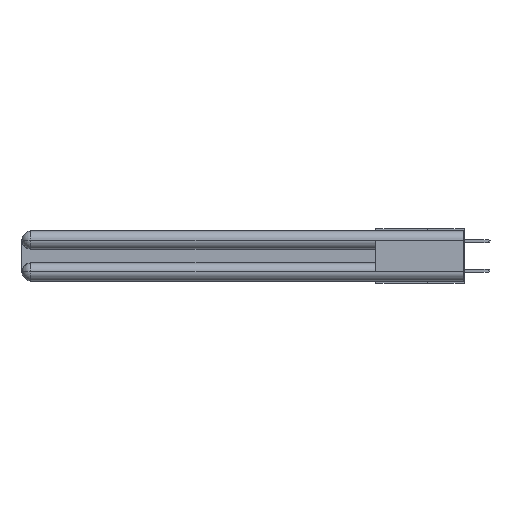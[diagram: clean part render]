
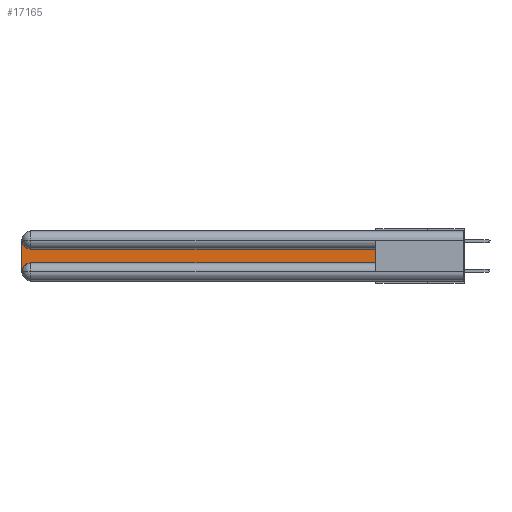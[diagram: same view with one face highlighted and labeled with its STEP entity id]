
A CAD part, left-side view. The second image highlights one B-rep face of the part: STEP entity #17165.
In plain terms, the highlighted planar face has unit normal (-1, 0, 0).
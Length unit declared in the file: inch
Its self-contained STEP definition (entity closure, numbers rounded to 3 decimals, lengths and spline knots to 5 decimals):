
#747 = CARTESIAN_POINT ( 'NONE',  ( 0.075, 0.6, -0.2175 ) ) ;
#974 = VERTEX_POINT ( 'NONE', #21450 ) ;
#1210 = EDGE_CURVE ( 'NONE', #27444, #25030, #19799, .T. ) ;
#1501 = VECTOR ( 'NONE', #4191, 39.37008 ) ;
#1812 = CARTESIAN_POINT ( 'NONE',  ( 0.075, 3., -0.2175 ) ) ;
#1838 = CARTESIAN_POINT ( 'NONE',  ( 0.075, 0.6, -0.2175 ) ) ;
#2228 = VERTEX_POINT ( 'NONE', #24825 ) ;
#2661 = AXIS2_PLACEMENT_3D ( 'NONE', #15143, #6917, #24907 ) ;
#3260 = DIRECTION ( 'NONE',  ( 0., -1., 0. ) ) ;
#4191 = DIRECTION ( 'NONE',  ( 0., 0., -1. ) ) ;
#4223 = AXIS2_PLACEMENT_3D ( 'NONE', #7172, #19726, #27407 ) ;
#4326 = DIRECTION ( 'NONE',  ( 0., 0., 1. ) ) ;
#5425 = LINE ( 'NONE', #747, #11995 ) ;
#5729 = VERTEX_POINT ( 'NONE', #16882 ) ;
#5844 = ORIENTED_EDGE ( 'NONE', *, *, #1210, .T. ) ;
#6917 = DIRECTION ( 'NONE',  ( 1., 0., 0. ) ) ;
#7108 = EDGE_CURVE ( 'NONE', #25030, #5729, #9244, .T. ) ;
#7115 = LINE ( 'NONE', #17999, #23766 ) ;
#7172 = CARTESIAN_POINT ( 'NONE',  ( 0.075, 2.94, -0.0625 ) ) ;
#7848 = ORIENTED_EDGE ( 'NONE', *, *, #7108, .T. ) ;
#9244 = LINE ( 'NONE', #1812, #1501 ) ;
#9926 = ORIENTED_EDGE ( 'NONE', *, *, #19252, .T. ) ;
#11804 = ORIENTED_EDGE ( 'NONE', *, *, #27082, .T. ) ;
#11995 = VECTOR ( 'NONE', #3260, 39.37008 ) ;
#13888 = CARTESIAN_POINT ( 'NONE',  ( 0.075, 2.94, -0.2175 ) ) ;
#14160 = DIRECTION ( 'NONE',  ( 1., 0., 0. ) ) ;
#15131 = VECTOR ( 'NONE', #4326, 39.37008 ) ;
#15143 = CARTESIAN_POINT ( 'NONE',  ( 0.075, 2.94, -0.2775 ) ) ;
#15382 = VERTEX_POINT ( 'NONE', #13888 ) ;
#16882 = CARTESIAN_POINT ( 'NONE',  ( 0.075, 3., -0.2775 ) ) ;
#17165 = ADVANCED_FACE ( 'NONE', ( #28201 ), #31717, .F. ) ;
#17275 = CARTESIAN_POINT ( 'NONE',  ( 0.075, 3., -0.0625 ) ) ;
#17999 = CARTESIAN_POINT ( 'NONE',  ( 0.075, 0.6, -0.1225 ) ) ;
#18588 = ORIENTED_EDGE ( 'NONE', *, *, #30420, .T. ) ;
#19252 = EDGE_CURVE ( 'NONE', #2228, #27444, #7115, .T. ) ;
#19726 = DIRECTION ( 'NONE',  ( 1., 0., 0. ) ) ;
#19799 = CIRCLE ( 'NONE', #4223, 0.06 ) ;
#20093 = ORIENTED_EDGE ( 'NONE', *, *, #23962, .T. ) ;
#20283 = DIRECTION ( 'NONE',  ( 0., 1., 0. ) ) ;
#20817 = CARTESIAN_POINT ( 'NONE',  ( 0.075, 2.94, -0.1225 ) ) ;
#21071 = EDGE_LOOP ( 'NONE', ( #9926, #5844, #7848, #20093, #18588, #11804 ) ) ;
#21450 = CARTESIAN_POINT ( 'NONE',  ( 0.075, 0.6, -0.2175 ) ) ;
#22741 = CIRCLE ( 'NONE', #2661, 0.06 ) ;
#23766 = VECTOR ( 'NONE', #20283, 39.37008 ) ;
#23962 = EDGE_CURVE ( 'NONE', #5729, #15382, #22741, .T. ) ;
#24825 = CARTESIAN_POINT ( 'NONE',  ( 0.075, 0.6, -0.1225 ) ) ;
#24907 = DIRECTION ( 'NONE',  ( 0., 0., -1. ) ) ;
#25030 = VERTEX_POINT ( 'NONE', #17275 ) ;
#27082 = EDGE_CURVE ( 'NONE', #974, #2228, #27170, .T. ) ;
#27170 = LINE ( 'NONE', #1838, #15131 ) ;
#27407 = DIRECTION ( 'NONE',  ( 0., 0., -1. ) ) ;
#27444 = VERTEX_POINT ( 'NONE', #20817 ) ;
#28201 = FACE_OUTER_BOUND ( 'NONE', #21071, .T. ) ;
#29114 = CARTESIAN_POINT ( 'NONE',  ( 0.075, 3., -0.1225 ) ) ;
#29323 = AXIS2_PLACEMENT_3D ( 'NONE', #29114, #14160, #29336 ) ;
#29336 = DIRECTION ( 'NONE',  ( 0., 0., -1. ) ) ;
#30420 = EDGE_CURVE ( 'NONE', #15382, #974, #5425, .T. ) ;
#31717 = PLANE ( 'NONE',  #29323 ) ;
